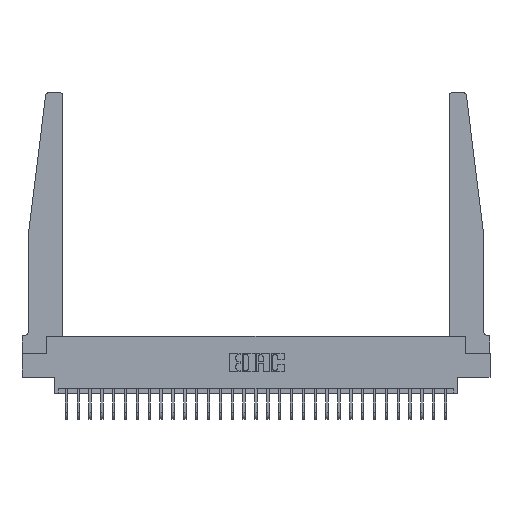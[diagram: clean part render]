
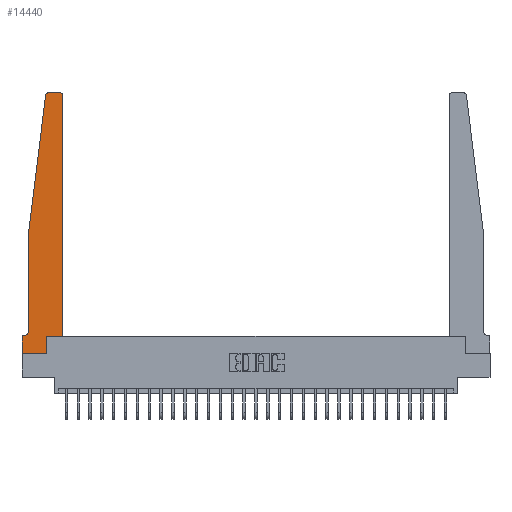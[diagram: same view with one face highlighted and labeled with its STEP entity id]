
A CAD part, top view. The second image highlights one B-rep face of the part: STEP entity #14440.
In plain terms, the highlighted planar face has unit normal (0, 0, 1).
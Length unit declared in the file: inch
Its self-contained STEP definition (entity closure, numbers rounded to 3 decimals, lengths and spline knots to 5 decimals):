
#342 = CARTESIAN_POINT ( 'NONE',  ( 0.2605, 0.18, 0.37 ) ) ;
#456 = VERTEX_POINT ( 'NONE', #22445 ) ;
#715 = CIRCLE ( 'NONE', #25333, 0.05 ) ;
#1141 = EDGE_CURVE ( 'NONE', #2709, #19765, #27358, .T. ) ;
#1273 = LINE ( 'NONE', #14873, #10174 ) ;
#1315 = DIRECTION ( 'NONE',  ( -1., 0., 0. ) ) ;
#1734 = EDGE_CURVE ( 'NONE', #10377, #15482, #21799, .T. ) ;
#1882 = EDGE_CURVE ( 'NONE', #14951, #7041, #20280, .T. ) ;
#1961 = CARTESIAN_POINT ( 'NONE',  ( 0.065, 1.25, 0.37 ) ) ;
#2198 = VERTEX_POINT ( 'NONE', #12978 ) ;
#2238 = CARTESIAN_POINT ( 'NONE',  ( 0.425, 0.18, 0.37 ) ) ;
#2242 = VECTOR ( 'NONE', #16713, 39.37008 ) ;
#2709 = VERTEX_POINT ( 'NONE', #342 ) ;
#3958 = EDGE_LOOP ( 'NONE', ( #29109, #21379, #18077, #18966, #14077, #14388, #14579, #13495, #16044, #22942, #18251, #10006 ) ) ;
#4500 = DIRECTION ( 'NONE',  ( 1., 0., 0. ) ) ;
#4518 = DIRECTION ( 'NONE',  ( 1., 0., 0. ) ) ;
#4656 = VECTOR ( 'NONE', #21389, 39.37008 ) ;
#5053 = CARTESIAN_POINT ( 'NONE',  ( 0.2605, 0.18, 0.37 ) ) ;
#5078 = CARTESIAN_POINT ( 'NONE',  ( 0.425, 0.18, 0.37 ) ) ;
#6411 = VECTOR ( 'NONE', #14839, 39.37008 ) ;
#6623 = DIRECTION ( 'NONE',  ( 0., 0., -1. ) ) ;
#7041 = VERTEX_POINT ( 'NONE', #1961 ) ;
#7217 = EDGE_CURVE ( 'NONE', #456, #14951, #8681, .T. ) ;
#7219 = AXIS2_PLACEMENT_3D ( 'NONE', #21455, #18876, #16601 ) ;
#7627 = DIRECTION ( 'NONE',  ( -1., 0., 0. ) ) ;
#7879 = CARTESIAN_POINT ( 'NONE',  ( 0.065, 0.2375, 0.37 ) ) ;
#8020 = VERTEX_POINT ( 'NONE', #18207 ) ;
#8046 = CARTESIAN_POINT ( 'NONE',  ( 0., 0., 0.37 ) ) ;
#8235 = EDGE_CURVE ( 'NONE', #8020, #456, #1273, .T. ) ;
#8681 = CIRCLE ( 'NONE', #7219, 0.03 ) ;
#9615 = CARTESIAN_POINT ( 'NONE',  ( 0., 0., 0.37 ) ) ;
#9950 = CARTESIAN_POINT ( 'NONE',  ( 0.24675, 2.72367, 0.37 ) ) ;
#10006 = ORIENTED_EDGE ( 'NONE', *, *, #27834, .T. ) ;
#10007 = LINE ( 'NONE', #10302, #6411 ) ;
#10174 = VECTOR ( 'NONE', #7627, 39.37008 ) ;
#10302 = CARTESIAN_POINT ( 'NONE',  ( 0., 0., 0.37 ) ) ;
#10303 = DIRECTION ( 'NONE',  ( 0., -1., 0. ) ) ;
#10377 = VERTEX_POINT ( 'NONE', #18625 ) ;
#10576 = CIRCLE ( 'NONE', #11040, 0.03 ) ;
#10585 = EDGE_CURVE ( 'NONE', #15482, #24355, #10007, .T. ) ;
#11040 = AXIS2_PLACEMENT_3D ( 'NONE', #13891, #15722, #4518 ) ;
#11326 = EDGE_CURVE ( 'NONE', #7041, #24775, #13233, .T. ) ;
#11955 = DIRECTION ( 'NONE',  ( 1., 0., 0. ) ) ;
#12978 = CARTESIAN_POINT ( 'NONE',  ( 0.015, 0.1875, 0.37 ) ) ;
#13070 = VECTOR ( 'NONE', #18212, 39.37008 ) ;
#13233 = LINE ( 'NONE', #25176, #13070 ) ;
#13495 = ORIENTED_EDGE ( 'NONE', *, *, #10585, .T. ) ;
#13891 = CARTESIAN_POINT ( 'NONE',  ( 0.395, 2.72, 0.37 ) ) ;
#14077 = ORIENTED_EDGE ( 'NONE', *, *, #21054, .T. ) ;
#14388 = ORIENTED_EDGE ( 'NONE', *, *, #29733, .T. ) ;
#14440 = ADVANCED_FACE ( 'NONE', ( #21491 ), #16634, .T. ) ;
#14579 = ORIENTED_EDGE ( 'NONE', *, *, #1734, .T. ) ;
#14839 = DIRECTION ( 'NONE',  ( 1., 0., 0. ) ) ;
#14873 = CARTESIAN_POINT ( 'NONE',  ( 0.25, 2.75, 0.37 ) ) ;
#14951 = VERTEX_POINT ( 'NONE', #9950 ) ;
#15482 = VERTEX_POINT ( 'NONE', #9615 ) ;
#15700 = VERTEX_POINT ( 'NONE', #22608 ) ;
#15722 = DIRECTION ( 'NONE',  ( 0., 0., 1. ) ) ;
#16044 = ORIENTED_EDGE ( 'NONE', *, *, #17236, .T. ) ;
#16601 = DIRECTION ( 'NONE',  ( 1., 0., 0. ) ) ;
#16628 = AXIS2_PLACEMENT_3D ( 'NONE', #23289, #28001, #11955 ) ;
#16634 = PLANE ( 'NONE',  #16628 ) ;
#16713 = DIRECTION ( 'NONE',  ( 0., 1., 0. ) ) ;
#17236 = EDGE_CURVE ( 'NONE', #24355, #2709, #23337, .T. ) ;
#18077 = ORIENTED_EDGE ( 'NONE', *, *, #1882, .T. ) ;
#18207 = CARTESIAN_POINT ( 'NONE',  ( 0.395, 2.75, 0.37 ) ) ;
#18212 = DIRECTION ( 'NONE',  ( 0., -1., 0. ) ) ;
#18251 = ORIENTED_EDGE ( 'NONE', *, *, #23623, .T. ) ;
#18625 = CARTESIAN_POINT ( 'NONE',  ( 0., 0.1875, 0.37 ) ) ;
#18876 = DIRECTION ( 'NONE',  ( 0., 0., 1. ) ) ;
#18966 = ORIENTED_EDGE ( 'NONE', *, *, #11326, .T. ) ;
#19604 = CARTESIAN_POINT ( 'NONE',  ( 0.065, 0.1875, 0.37 ) ) ;
#19765 = VERTEX_POINT ( 'NONE', #25051 ) ;
#20090 = CARTESIAN_POINT ( 'NONE',  ( 0.015, 0.2375, 0.37 ) ) ;
#20280 = LINE ( 'NONE', #29514, #20632 ) ;
#20632 = VECTOR ( 'NONE', #22689, 39.37008 ) ;
#21054 = EDGE_CURVE ( 'NONE', #24775, #2198, #715, .T. ) ;
#21379 = ORIENTED_EDGE ( 'NONE', *, *, #7217, .T. ) ;
#21389 = DIRECTION ( 'NONE',  ( 0., 1., 0. ) ) ;
#21455 = CARTESIAN_POINT ( 'NONE',  ( 0.27653, 2.72, 0.37 ) ) ;
#21491 = FACE_OUTER_BOUND ( 'NONE', #3958, .T. ) ;
#21799 = LINE ( 'NONE', #8046, #29807 ) ;
#22130 = CARTESIAN_POINT ( 'NONE',  ( 0.2605, 0., 0.37 ) ) ;
#22445 = CARTESIAN_POINT ( 'NONE',  ( 0.27653, 2.75, 0.37 ) ) ;
#22608 = CARTESIAN_POINT ( 'NONE',  ( 0.425, 2.72, 0.37 ) ) ;
#22689 = DIRECTION ( 'NONE',  ( -0.122, -0.992, 0. ) ) ;
#22942 = ORIENTED_EDGE ( 'NONE', *, *, #1141, .T. ) ;
#23289 = CARTESIAN_POINT ( 'NONE',  ( 0., 0.1875, 0.37 ) ) ;
#23337 = LINE ( 'NONE', #5053, #4656 ) ;
#23623 = EDGE_CURVE ( 'NONE', #19765, #15700, #28378, .T. ) ;
#23683 = VECTOR ( 'NONE', #1315, 39.37008 ) ;
#24355 = VERTEX_POINT ( 'NONE', #22130 ) ;
#24775 = VERTEX_POINT ( 'NONE', #7879 ) ;
#25051 = CARTESIAN_POINT ( 'NONE',  ( 0.425, 0.18, 0.37 ) ) ;
#25176 = CARTESIAN_POINT ( 'NONE',  ( 0.065, 1.25, 0.37 ) ) ;
#25208 = DIRECTION ( 'NONE',  ( -1., 0., 0. ) ) ;
#25333 = AXIS2_PLACEMENT_3D ( 'NONE', #20090, #6623, #25208 ) ;
#26859 = LINE ( 'NONE', #19604, #23683 ) ;
#27214 = VECTOR ( 'NONE', #4500, 39.37008 ) ;
#27358 = LINE ( 'NONE', #2238, #27214 ) ;
#27834 = EDGE_CURVE ( 'NONE', #15700, #8020, #10576, .T. ) ;
#28001 = DIRECTION ( 'NONE',  ( 0., 0., 1. ) ) ;
#28378 = LINE ( 'NONE', #5078, #2242 ) ;
#29109 = ORIENTED_EDGE ( 'NONE', *, *, #8235, .T. ) ;
#29514 = CARTESIAN_POINT ( 'NONE',  ( 0.065, 1.25, 0.37 ) ) ;
#29733 = EDGE_CURVE ( 'NONE', #2198, #10377, #26859, .T. ) ;
#29807 = VECTOR ( 'NONE', #10303, 39.37008 ) ;
